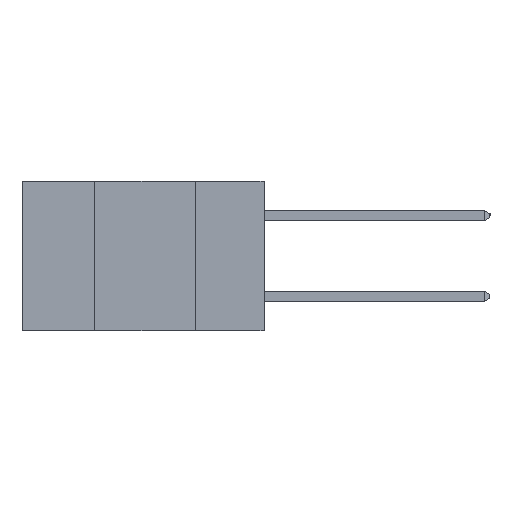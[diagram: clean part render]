
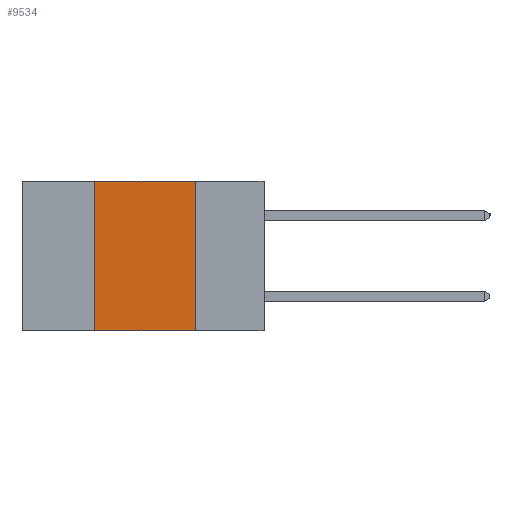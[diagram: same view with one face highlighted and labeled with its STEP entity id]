
A CAD part, left-side view. The second image highlights one B-rep face of the part: STEP entity #9534.
In plain terms, the highlighted planar face has unit normal (-1, 0, 0).
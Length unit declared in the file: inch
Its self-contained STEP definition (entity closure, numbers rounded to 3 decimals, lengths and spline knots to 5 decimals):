
#311 = DIRECTION ( 'NONE',  ( 0., -1., 0. ) ) ;
#332 = CARTESIAN_POINT ( 'NONE',  ( 0., 0.6, 0. ) ) ;
#925 = CARTESIAN_POINT ( 'NONE',  ( 0., 0.42, 0. ) ) ;
#1277 = CARTESIAN_POINT ( 'NONE',  ( 0., 0.17, 0. ) ) ;
#1351 = VERTEX_POINT ( 'NONE', #925 ) ;
#1625 = VERTEX_POINT ( 'NONE', #4706 ) ;
#2138 = LINE ( 'NONE', #3068, #4295 ) ;
#2161 = PLANE ( 'NONE',  #9426 ) ;
#2595 = EDGE_CURVE ( 'NONE', #1351, #11901, #11563, .T. ) ;
#3068 = CARTESIAN_POINT ( 'NONE',  ( 0., 0.42, 0. ) ) ;
#3721 = LINE ( 'NONE', #6477, #8350 ) ;
#3810 = ORIENTED_EDGE ( 'NONE', *, *, #5529, .F. ) ;
#4005 = DIRECTION ( 'NONE',  ( 0., 0., -1. ) ) ;
#4072 = DIRECTION ( 'NONE',  ( 0., -1., 0. ) ) ;
#4295 = VECTOR ( 'NONE', #10152, 39.37008 ) ;
#4571 = VECTOR ( 'NONE', #7380, 39.37008 ) ;
#4706 = CARTESIAN_POINT ( 'NONE',  ( 0., 0.42, -0.37 ) ) ;
#4731 = CARTESIAN_POINT ( 'NONE',  ( 0., 0.17, -0.37 ) ) ;
#5529 = EDGE_CURVE ( 'NONE', #11901, #9409, #9560, .T. ) ;
#5562 = EDGE_CURVE ( 'NONE', #1625, #1351, #2138, .T. ) ;
#5642 = EDGE_CURVE ( 'NONE', #1625, #9409, #3721, .T. ) ;
#6477 = CARTESIAN_POINT ( 'NONE',  ( 0., 0.6, -0.37 ) ) ;
#6616 = ORIENTED_EDGE ( 'NONE', *, *, #5562, .F. ) ;
#6956 = VECTOR ( 'NONE', #311, 39.37008 ) ;
#7380 = DIRECTION ( 'NONE',  ( 0., 0., -1. ) ) ;
#8309 = CARTESIAN_POINT ( 'NONE',  ( 0., 0.17, 0. ) ) ;
#8350 = VECTOR ( 'NONE', #4072, 39.37008 ) ;
#8630 = EDGE_LOOP ( 'NONE', ( #3810, #11194, #6616, #11478 ) ) ;
#8646 = CARTESIAN_POINT ( 'NONE',  ( 0., 0.6, 0. ) ) ;
#9409 = VERTEX_POINT ( 'NONE', #4731 ) ;
#9426 = AXIS2_PLACEMENT_3D ( 'NONE', #8646, #9602, #4005 ) ;
#9534 = ADVANCED_FACE ( 'NONE', ( #11037 ), #2161, .F. ) ;
#9560 = LINE ( 'NONE', #1277, #4571 ) ;
#9602 = DIRECTION ( 'NONE',  ( 1., 0., 0. ) ) ;
#10152 = DIRECTION ( 'NONE',  ( 0., 0., 1. ) ) ;
#11037 = FACE_OUTER_BOUND ( 'NONE', #8630, .T. ) ;
#11194 = ORIENTED_EDGE ( 'NONE', *, *, #2595, .F. ) ;
#11478 = ORIENTED_EDGE ( 'NONE', *, *, #5642, .T. ) ;
#11563 = LINE ( 'NONE', #332, #6956 ) ;
#11901 = VERTEX_POINT ( 'NONE', #8309 ) ;
